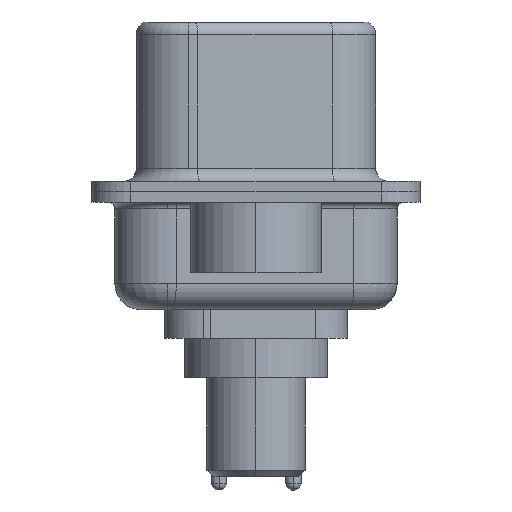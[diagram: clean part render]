
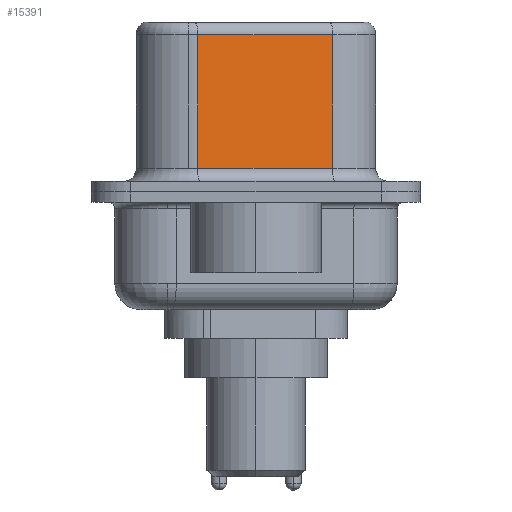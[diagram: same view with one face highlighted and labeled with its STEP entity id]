
A CAD part, left-side view. The second image highlights one B-rep face of the part: STEP entity #15391.
In plain terms, the highlighted planar face has unit normal (-0.985, -0.174, 0).
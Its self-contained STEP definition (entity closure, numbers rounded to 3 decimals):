
#789 = ORIENTED_EDGE ( 'NONE', *, *, #17663, .T. ) ;
#951 = DIRECTION ( 'NONE',  ( -0.174, 0.985, 0. ) ) ;
#1036 = CARTESIAN_POINT ( 'NONE',  ( 4.585, -2.927, 6.02 ) ) ;
#1040 = ORIENTED_EDGE ( 'NONE', *, *, #8151, .F. ) ;
#1114 = VECTOR ( 'NONE', #12618, 1000. ) ;
#1375 = AXIS2_PLACEMENT_3D ( 'NONE', #6732, #20576, #18651 ) ;
#1797 = CARTESIAN_POINT ( 'NONE',  ( 3.675, 2.233, 0.9 ) ) ;
#5919 = LINE ( 'NONE', #14637, #1114 ) ;
#6005 = VECTOR ( 'NONE', #9815, 1000. ) ;
#6289 = LINE ( 'NONE', #19961, #18092 ) ;
#6732 = CARTESIAN_POINT ( 'NONE',  ( 4.585, -2.927, 6.52 ) ) ;
#6844 = EDGE_CURVE ( 'NONE', #18098, #17038, #6289, .T. ) ;
#7574 = ORIENTED_EDGE ( 'NONE', *, *, #19398, .T. ) ;
#8151 = EDGE_CURVE ( 'NONE', #18098, #20089, #11400, .T. ) ;
#9194 = LINE ( 'NONE', #21586, #6005 ) ;
#9351 = CARTESIAN_POINT ( 'NONE',  ( 3.675, 2.233, 6.02 ) ) ;
#9815 = DIRECTION ( 'NONE',  ( 0., 0., -1. ) ) ;
#11400 = LINE ( 'NONE', #11563, #18387 ) ;
#11563 = CARTESIAN_POINT ( 'NONE',  ( 4.585, -2.927, 6.52 ) ) ;
#12618 = DIRECTION ( 'NONE',  ( 0.174, -0.985, 0. ) ) ;
#13527 = PLANE ( 'NONE',  #1375 ) ;
#14637 = CARTESIAN_POINT ( 'NONE',  ( 4.585, -2.927, 0.9 ) ) ;
#14879 = FACE_OUTER_BOUND ( 'NONE', #17526, .T. ) ;
#15204 = CARTESIAN_POINT ( 'NONE',  ( 4.585, -2.927, 0.9 ) ) ;
#15391 = ADVANCED_FACE ( 'NONE', ( #14879 ), #13527, .F. ) ;
#16756 = DIRECTION ( 'NONE',  ( 0., 0., -1. ) ) ;
#17038 = VERTEX_POINT ( 'NONE', #9351 ) ;
#17526 = EDGE_LOOP ( 'NONE', ( #1040, #17654, #7574, #789 ) ) ;
#17654 = ORIENTED_EDGE ( 'NONE', *, *, #6844, .T. ) ;
#17663 = EDGE_CURVE ( 'NONE', #18600, #20089, #5919, .T. ) ;
#18092 = VECTOR ( 'NONE', #951, 1000. ) ;
#18098 = VERTEX_POINT ( 'NONE', #1036 ) ;
#18387 = VECTOR ( 'NONE', #16756, 1000. ) ;
#18600 = VERTEX_POINT ( 'NONE', #1797 ) ;
#18651 = DIRECTION ( 'NONE',  ( -0.174, 0.985, 0. ) ) ;
#19398 = EDGE_CURVE ( 'NONE', #17038, #18600, #9194, .T. ) ;
#19961 = CARTESIAN_POINT ( 'NONE',  ( 4.585, -2.927, 6.02 ) ) ;
#20089 = VERTEX_POINT ( 'NONE', #15204 ) ;
#20576 = DIRECTION ( 'NONE',  ( 0.985, 0.174, 0. ) ) ;
#21586 = CARTESIAN_POINT ( 'NONE',  ( 3.675, 2.233, 6.52 ) ) ;
